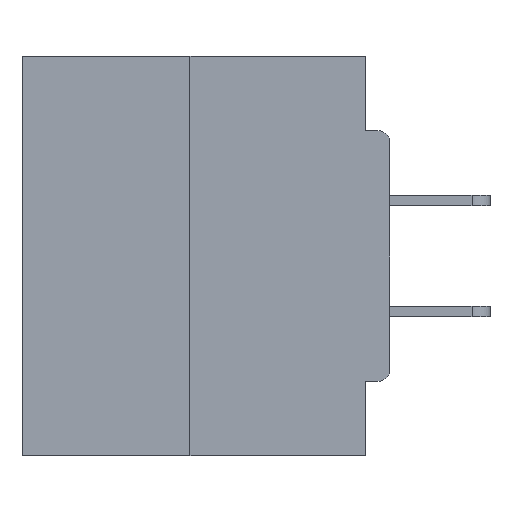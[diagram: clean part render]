
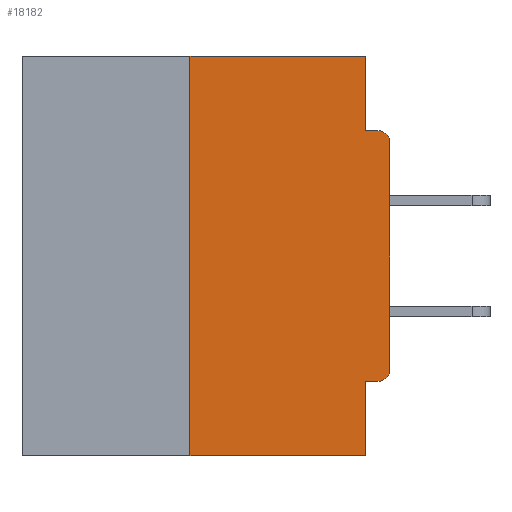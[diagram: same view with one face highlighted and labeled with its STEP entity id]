
A CAD part, left-side view. The second image highlights one B-rep face of the part: STEP entity #18182.
In plain terms, the highlighted planar face has unit normal (-1, 0, 0).
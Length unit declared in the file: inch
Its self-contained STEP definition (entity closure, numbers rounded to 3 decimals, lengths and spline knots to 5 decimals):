
#1118 = ORIENTED_EDGE ( 'NONE', *, *, #32332, .F. ) ;
#1879 = ORIENTED_EDGE ( 'NONE', *, *, #15120, .T. ) ;
#2033 = ORIENTED_EDGE ( 'NONE', *, *, #28273, .T. ) ;
#2052 = DIRECTION ( 'NONE',  ( -1., 0., 0. ) ) ;
#2974 = LINE ( 'NONE', #24232, #14761 ) ;
#3012 = CARTESIAN_POINT ( 'NONE',  ( 0., 0.031, -0.0935 ) ) ;
#3696 = FACE_OUTER_BOUND ( 'NONE', #6619, .T. ) ;
#3962 = VERTEX_POINT ( 'NONE', #32808 ) ;
#4255 = VECTOR ( 'NONE', #27769, 39.37008 ) ;
#5199 = EDGE_CURVE ( 'NONE', #9179, #3962, #2974, .T. ) ;
#5907 = LINE ( 'NONE', #10765, #20022 ) ;
#6318 = CARTESIAN_POINT ( 'NONE',  ( 0., 0.46, -0.5 ) ) ;
#6619 = EDGE_LOOP ( 'NONE', ( #14607, #8678, #14818, #34800, #8699, #1879, #35587, #2033, #32684, #1118 ) ) ;
#6745 = CARTESIAN_POINT ( 'NONE',  ( 0., 0.031, 0. ) ) ;
#6879 = VERTEX_POINT ( 'NONE', #10601 ) ;
#7211 = CIRCLE ( 'NONE', #27978, 0.015 ) ;
#7253 = CARTESIAN_POINT ( 'NONE',  ( 0., 0.015, -0.0935 ) ) ;
#7361 = LINE ( 'NONE', #6318, #10193 ) ;
#7737 = EDGE_CURVE ( 'NONE', #23050, #33495, #21835, .T. ) ;
#7842 = DIRECTION ( 'NONE',  ( 0., -1., 0. ) ) ;
#8153 = DIRECTION ( 'NONE',  ( 0., -1., 0. ) ) ;
#8580 = DIRECTION ( 'NONE',  ( -1., 0., 0. ) ) ;
#8678 = ORIENTED_EDGE ( 'NONE', *, *, #17233, .F. ) ;
#8699 = ORIENTED_EDGE ( 'NONE', *, *, #14136, .F. ) ;
#9179 = VERTEX_POINT ( 'NONE', #32880 ) ;
#9350 = DIRECTION ( 'NONE',  ( 0., 0., -1. ) ) ;
#9778 = DIRECTION ( 'NONE',  ( 0., 0., -1. ) ) ;
#10193 = VECTOR ( 'NONE', #7842, 39.37008 ) ;
#10322 = LINE ( 'NONE', #36644, #4255 ) ;
#10601 = CARTESIAN_POINT ( 'NONE',  ( 0., 0.031, 0. ) ) ;
#10765 = CARTESIAN_POINT ( 'NONE',  ( 0., 0., -0.4065 ) ) ;
#10859 = VECTOR ( 'NONE', #34198, 39.37008 ) ;
#11765 = CARTESIAN_POINT ( 'NONE',  ( 0., 0., -0.0935 ) ) ;
#11895 = AXIS2_PLACEMENT_3D ( 'NONE', #16756, #35096, #37843 ) ;
#11988 = VERTEX_POINT ( 'NONE', #21564 ) ;
#13425 = VERTEX_POINT ( 'NONE', #29145 ) ;
#14136 = EDGE_CURVE ( 'NONE', #31632, #9179, #5907, .T. ) ;
#14607 = ORIENTED_EDGE ( 'NONE', *, *, #18968, .F. ) ;
#14761 = VECTOR ( 'NONE', #9350, 39.37008 ) ;
#14818 = ORIENTED_EDGE ( 'NONE', *, *, #38439, .T. ) ;
#15120 = EDGE_CURVE ( 'NONE', #31632, #38182, #7211, .T. ) ;
#16756 = CARTESIAN_POINT ( 'NONE',  ( 0., 0.46, 0. ) ) ;
#17187 = AXIS2_PLACEMENT_3D ( 'NONE', #17901, #8580, #36008 ) ;
#17233 = EDGE_CURVE ( 'NONE', #20541, #13425, #10322, .T. ) ;
#17901 = CARTESIAN_POINT ( 'NONE',  ( 0., 0.015, -0.1085 ) ) ;
#18182 = ADVANCED_FACE ( 'NONE', ( #3696 ), #34837, .F. ) ;
#18968 = EDGE_CURVE ( 'NONE', #13425, #6879, #21542, .T. ) ;
#19353 = CARTESIAN_POINT ( 'NONE',  ( 0., 0.015, -0.4065 ) ) ;
#19641 = VECTOR ( 'NONE', #8153, 39.37008 ) ;
#19767 = CARTESIAN_POINT ( 'NONE',  ( 0., 0.25, -0.5 ) ) ;
#20022 = VECTOR ( 'NONE', #31570, 39.37008 ) ;
#20541 = VERTEX_POINT ( 'NONE', #19767 ) ;
#21542 = LINE ( 'NONE', #35444, #19641 ) ;
#21564 = CARTESIAN_POINT ( 'NONE',  ( 0., 0., -0.1085 ) ) ;
#21677 = CARTESIAN_POINT ( 'NONE',  ( 0., 0., 0. ) ) ;
#21835 = LINE ( 'NONE', #11765, #22787 ) ;
#22787 = VECTOR ( 'NONE', #27041, 39.37008 ) ;
#23050 = VERTEX_POINT ( 'NONE', #3012 ) ;
#23407 = CARTESIAN_POINT ( 'NONE',  ( 0., 0.015, -0.3915 ) ) ;
#23920 = VECTOR ( 'NONE', #9778, 39.37008 ) ;
#24232 = CARTESIAN_POINT ( 'NONE',  ( 0., 0.031, -0.5 ) ) ;
#24346 = CARTESIAN_POINT ( 'NONE',  ( 0., 0., -0.3915 ) ) ;
#27041 = DIRECTION ( 'NONE',  ( 0., -1., 0. ) ) ;
#27769 = DIRECTION ( 'NONE',  ( 0., 0., 1. ) ) ;
#27978 = AXIS2_PLACEMENT_3D ( 'NONE', #23407, #2052, #35677 ) ;
#28273 = EDGE_CURVE ( 'NONE', #11988, #33495, #35429, .T. ) ;
#28562 = EDGE_CURVE ( 'NONE', #38182, #11988, #36807, .T. ) ;
#29145 = CARTESIAN_POINT ( 'NONE',  ( 0., 0.25, 0. ) ) ;
#30044 = LINE ( 'NONE', #6745, #23920 ) ;
#31570 = DIRECTION ( 'NONE',  ( 0., 1., 0. ) ) ;
#31632 = VERTEX_POINT ( 'NONE', #19353 ) ;
#32332 = EDGE_CURVE ( 'NONE', #6879, #23050, #30044, .T. ) ;
#32684 = ORIENTED_EDGE ( 'NONE', *, *, #7737, .F. ) ;
#32808 = CARTESIAN_POINT ( 'NONE',  ( 0., 0.031, -0.5 ) ) ;
#32880 = CARTESIAN_POINT ( 'NONE',  ( 0., 0.031, -0.4065 ) ) ;
#33495 = VERTEX_POINT ( 'NONE', #7253 ) ;
#34198 = DIRECTION ( 'NONE',  ( 0., 0., 1. ) ) ;
#34800 = ORIENTED_EDGE ( 'NONE', *, *, #5199, .F. ) ;
#34837 = PLANE ( 'NONE',  #11895 ) ;
#35096 = DIRECTION ( 'NONE',  ( 1., 0., 0. ) ) ;
#35429 = CIRCLE ( 'NONE', #17187, 0.015 ) ;
#35444 = CARTESIAN_POINT ( 'NONE',  ( 0., 0.46, 0. ) ) ;
#35587 = ORIENTED_EDGE ( 'NONE', *, *, #28562, .T. ) ;
#35677 = DIRECTION ( 'NONE',  ( 0., 0., -1. ) ) ;
#36008 = DIRECTION ( 'NONE',  ( 0., 0., -1. ) ) ;
#36644 = CARTESIAN_POINT ( 'NONE',  ( 0., 0.25, 0. ) ) ;
#36807 = LINE ( 'NONE', #21677, #10859 ) ;
#37843 = DIRECTION ( 'NONE',  ( 0., 0., -1. ) ) ;
#38182 = VERTEX_POINT ( 'NONE', #24346 ) ;
#38439 = EDGE_CURVE ( 'NONE', #20541, #3962, #7361, .T. ) ;
